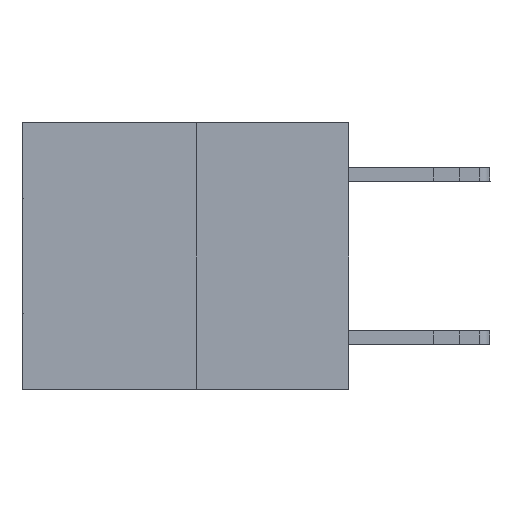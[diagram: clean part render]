
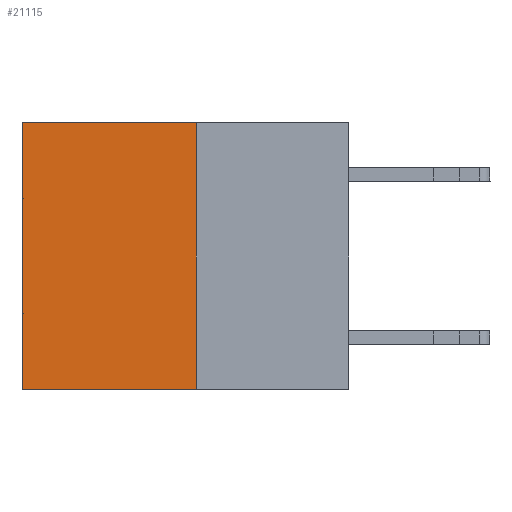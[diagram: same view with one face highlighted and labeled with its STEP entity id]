
A CAD part, left-side view. The second image highlights one B-rep face of the part: STEP entity #21115.
In plain terms, the highlighted planar face has unit normal (-1, 0, 0).
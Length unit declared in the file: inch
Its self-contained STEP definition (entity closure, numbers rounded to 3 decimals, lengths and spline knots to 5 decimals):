
#577 = CARTESIAN_POINT ( 'NONE',  ( 0.3165, 0.28, -0.49 ) ) ;
#1333 = CARTESIAN_POINT ( 'NONE',  ( 0.3165, 0.28, 0. ) ) ;
#1391 = AXIS2_PLACEMENT_3D ( 'NONE', #577, #19311, #25515 ) ;
#2311 = ORIENTED_EDGE ( 'NONE', *, *, #24544, .F. ) ;
#2648 = ORIENTED_EDGE ( 'NONE', *, *, #4992, .T. ) ;
#2677 = LINE ( 'NONE', #8824, #11756 ) ;
#4992 = EDGE_CURVE ( 'NONE', #27600, #13358, #20919, .T. ) ;
#5003 = VECTOR ( 'NONE', #23838, 39.37008 ) ;
#6170 = LINE ( 'NONE', #11080, #5003 ) ;
#6291 = EDGE_CURVE ( 'NONE', #22094, #29366, #2677, .T. ) ;
#8824 = CARTESIAN_POINT ( 'NONE',  ( 0.3165, 0.28, -0.49 ) ) ;
#9031 = DIRECTION ( 'NONE',  ( 0., 1., 0. ) ) ;
#9101 = LINE ( 'NONE', #23789, #11138 ) ;
#11080 = CARTESIAN_POINT ( 'NONE',  ( 0.3165, 0.6, -0.49 ) ) ;
#11138 = VECTOR ( 'NONE', #31003, 39.37008 ) ;
#11756 = VECTOR ( 'NONE', #9031, 39.37008 ) ;
#13358 = VERTEX_POINT ( 'NONE', #29057 ) ;
#17391 = DIRECTION ( 'NONE',  ( 0., 1., 0. ) ) ;
#17914 = EDGE_CURVE ( 'NONE', #13358, #29366, #6170, .T. ) ;
#18658 = ORIENTED_EDGE ( 'NONE', *, *, #17914, .T. ) ;
#19311 = DIRECTION ( 'NONE',  ( 1., 0., 0. ) ) ;
#20543 = CARTESIAN_POINT ( 'NONE',  ( 0.3165, 0.6, -0.49 ) ) ;
#20919 = LINE ( 'NONE', #32453, #22871 ) ;
#21115 = ADVANCED_FACE ( 'NONE', ( #29857 ), #28207, .F. ) ;
#22094 = VERTEX_POINT ( 'NONE', #23016 ) ;
#22871 = VECTOR ( 'NONE', #17391, 39.37008 ) ;
#22994 = ORIENTED_EDGE ( 'NONE', *, *, #6291, .F. ) ;
#23016 = CARTESIAN_POINT ( 'NONE',  ( 0.3165, 0.28, -0.49 ) ) ;
#23789 = CARTESIAN_POINT ( 'NONE',  ( 0.3165, 0.28, -0.49 ) ) ;
#23838 = DIRECTION ( 'NONE',  ( 0., 0., -1. ) ) ;
#24544 = EDGE_CURVE ( 'NONE', #27600, #22094, #9101, .T. ) ;
#25515 = DIRECTION ( 'NONE',  ( 0., 0., -1. ) ) ;
#27600 = VERTEX_POINT ( 'NONE', #1333 ) ;
#28207 = PLANE ( 'NONE',  #1391 ) ;
#29057 = CARTESIAN_POINT ( 'NONE',  ( 0.3165, 0.6, 0. ) ) ;
#29366 = VERTEX_POINT ( 'NONE', #20543 ) ;
#29857 = FACE_OUTER_BOUND ( 'NONE', #30540, .T. ) ;
#30540 = EDGE_LOOP ( 'NONE', ( #18658, #22994, #2311, #2648 ) ) ;
#31003 = DIRECTION ( 'NONE',  ( 0., 0., -1. ) ) ;
#32453 = CARTESIAN_POINT ( 'NONE',  ( 0.3165, 0.28, 0. ) ) ;
